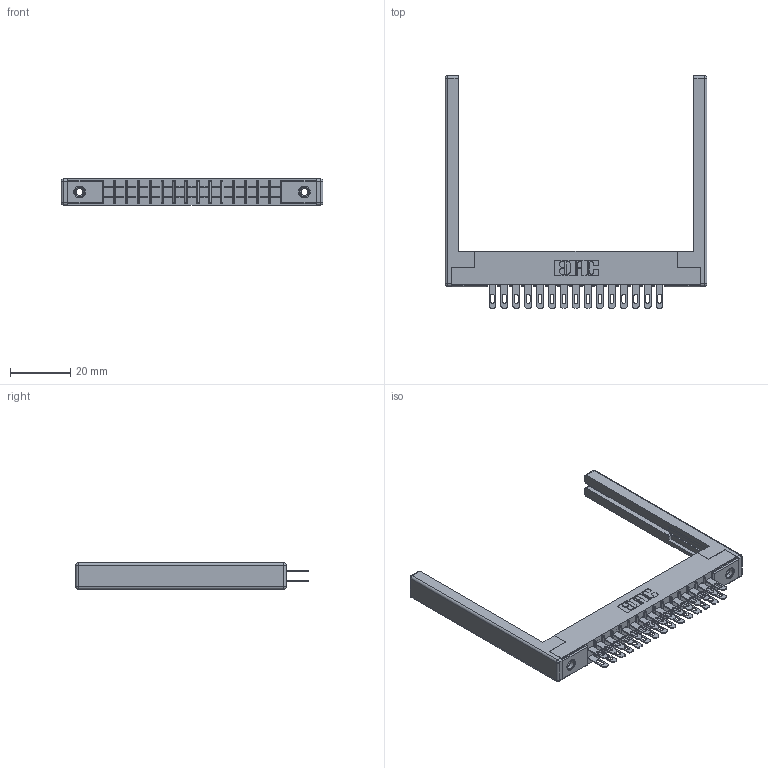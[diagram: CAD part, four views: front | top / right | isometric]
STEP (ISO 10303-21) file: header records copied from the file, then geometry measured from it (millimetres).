
FILE_DESCRIPTION (( 'STEP AP203' ), '1' );
FILE_NAME ('355-030-500-568.STEP', '2019-09-11T06:54:34', ( '' ), ( '' ), 'SwSTEP 2.0', 'SolidWorks 2016', '' );
FILE_SCHEMA (( 'CONFIG_CONTROL_DESIGN' ));
Length unit declared in the file: inch
Products named in the file (5): 345-250-001_345-250-001-102; 307-220-068; 305 Part_.156 Dia; 355-030-500-568; 305-290-001_500
Assembly tree (35 placements, depth 2):
  355-030-500-568
    305 Part_.156 Dia
    305-290-001_500  x30
    345-250-001_345-250-001-102  x2
    307-220-068  x2
Bounding box: 86.87 x 77.14 x 8.71 mm (x, y, z)
Volume: 9911.5 mm3; surface area: 14708 mm2
Topology: 35 solids, 35 shells, 1770 faces, 5011 edges, 3238 vertices
Faces by surface type: plane 996, cylinder 690, sphere 68, cone 12, torus 4
Entity records: 22309 total; most frequent: CARTESIAN_POINT 3664, ORIENTED_EDGE 3624, DIRECTION 3588, EDGE_CURVE 1812, VECTOR 1424, LINE 1424, VERTEX_POINT 1158, AXIS2_PLACEMENT_3D 1082
